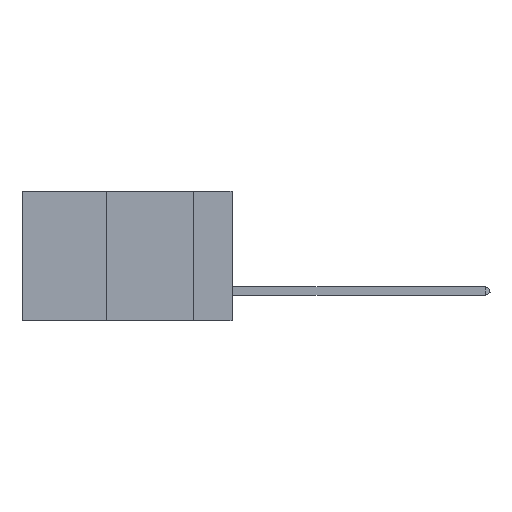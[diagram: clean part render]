
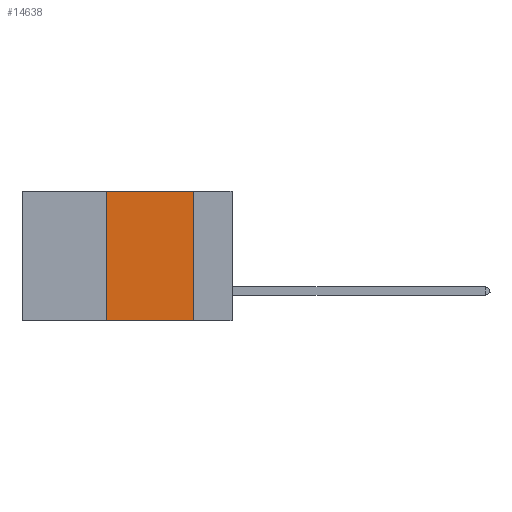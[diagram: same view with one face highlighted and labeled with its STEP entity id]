
A CAD part, left-side view. The second image highlights one B-rep face of the part: STEP entity #14638.
In plain terms, the highlighted planar face has unit normal (-1, 0, 0).
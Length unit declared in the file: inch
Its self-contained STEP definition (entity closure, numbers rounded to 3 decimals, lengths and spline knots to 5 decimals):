
#167 = LINE ( 'NONE', #2284, #14382 ) ;
#254 = CARTESIAN_POINT ( 'NONE',  ( 0., 0.6, -0.37 ) ) ;
#485 = CARTESIAN_POINT ( 'NONE',  ( 0., 0.36, -0.37 ) ) ;
#1441 = LINE ( 'NONE', #4855, #25504 ) ;
#1852 = CARTESIAN_POINT ( 'NONE',  ( 0., 0.36, 0. ) ) ;
#2132 = DIRECTION ( 'NONE',  ( 0., 0., -1. ) ) ;
#2284 = CARTESIAN_POINT ( 'NONE',  ( 0., 0.6, 0. ) ) ;
#3124 = CARTESIAN_POINT ( 'NONE',  ( 0., 0.11, -0.37 ) ) ;
#4855 = CARTESIAN_POINT ( 'NONE',  ( 0., 0.11, 0. ) ) ;
#5249 = VECTOR ( 'NONE', #10063, 39.37008 ) ;
#6027 = CARTESIAN_POINT ( 'NONE',  ( 0., 0.6, 0. ) ) ;
#8332 = CARTESIAN_POINT ( 'NONE',  ( 0., 0.36, 0. ) ) ;
#8380 = DIRECTION ( 'NONE',  ( 0., -1., 0. ) ) ;
#9796 = VERTEX_POINT ( 'NONE', #3124 ) ;
#10063 = DIRECTION ( 'NONE',  ( 0., -1., 0. ) ) ;
#11246 = LINE ( 'NONE', #254, #5249 ) ;
#12029 = DIRECTION ( 'NONE',  ( 1., 0., 0. ) ) ;
#12649 = CARTESIAN_POINT ( 'NONE',  ( 0., 0.11, 0. ) ) ;
#12844 = ORIENTED_EDGE ( 'NONE', *, *, #22261, .F. ) ;
#13395 = ORIENTED_EDGE ( 'NONE', *, *, #15259, .T. ) ;
#13833 = VECTOR ( 'NONE', #23758, 39.37008 ) ;
#14069 = VERTEX_POINT ( 'NONE', #485 ) ;
#14382 = VECTOR ( 'NONE', #8380, 39.37008 ) ;
#14638 = ADVANCED_FACE ( 'NONE', ( #20447 ), #16216, .F. ) ;
#15221 = EDGE_CURVE ( 'NONE', #14069, #20776, #16050, .T. ) ;
#15259 = EDGE_CURVE ( 'NONE', #14069, #9796, #11246, .T. ) ;
#15353 = EDGE_LOOP ( 'NONE', ( #12844, #25508, #15507, #13395 ) ) ;
#15507 = ORIENTED_EDGE ( 'NONE', *, *, #15221, .F. ) ;
#16050 = LINE ( 'NONE', #1852, #13833 ) ;
#16216 = PLANE ( 'NONE',  #22073 ) ;
#16613 = VERTEX_POINT ( 'NONE', #12649 ) ;
#20447 = FACE_OUTER_BOUND ( 'NONE', #15353, .T. ) ;
#20776 = VERTEX_POINT ( 'NONE', #8332 ) ;
#22073 = AXIS2_PLACEMENT_3D ( 'NONE', #6027, #12029, #2132 ) ;
#22261 = EDGE_CURVE ( 'NONE', #16613, #9796, #1441, .T. ) ;
#22983 = EDGE_CURVE ( 'NONE', #20776, #16613, #167, .T. ) ;
#23758 = DIRECTION ( 'NONE',  ( 0., 0., 1. ) ) ;
#25119 = DIRECTION ( 'NONE',  ( 0., 0., -1. ) ) ;
#25504 = VECTOR ( 'NONE', #25119, 39.37008 ) ;
#25508 = ORIENTED_EDGE ( 'NONE', *, *, #22983, .F. ) ;
